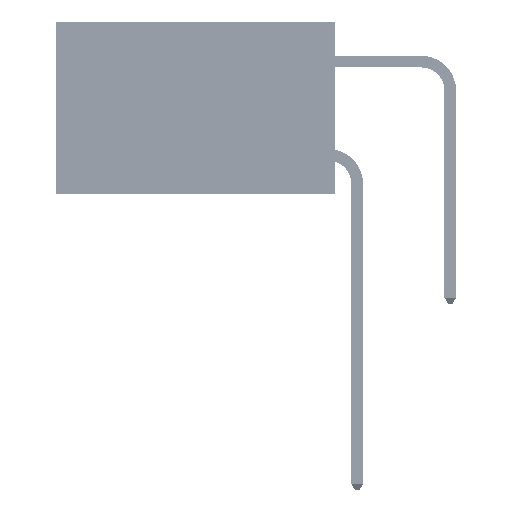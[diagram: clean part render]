
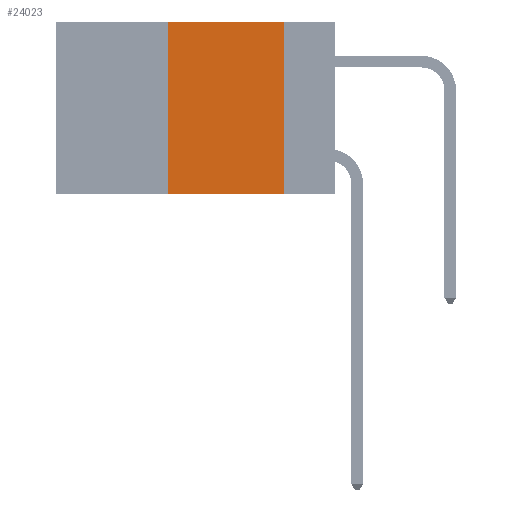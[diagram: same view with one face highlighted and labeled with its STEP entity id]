
A CAD part, left-side view. The second image highlights one B-rep face of the part: STEP entity #24023.
In plain terms, the highlighted planar face has unit normal (-1, 0, 0).
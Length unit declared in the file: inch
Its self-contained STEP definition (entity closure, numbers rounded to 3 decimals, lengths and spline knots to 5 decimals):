
#406 = CARTESIAN_POINT ( 'NONE',  ( 0., 0.11, -0.37 ) ) ;
#1248 = LINE ( 'NONE', #21266, #43485 ) ;
#2082 = EDGE_CURVE ( 'NONE', #16525, #44125, #23663, .T. ) ;
#4859 = VERTEX_POINT ( 'NONE', #8929 ) ;
#5444 = CARTESIAN_POINT ( 'NONE',  ( 0., 0.6, -0.37 ) ) ;
#6294 = VECTOR ( 'NONE', #39252, 39.37008 ) ;
#7403 = VECTOR ( 'NONE', #13469, 39.37008 ) ;
#8119 = ORIENTED_EDGE ( 'NONE', *, *, #2082, .F. ) ;
#8929 = CARTESIAN_POINT ( 'NONE',  ( 0., 0.36, -0.37 ) ) ;
#13469 = DIRECTION ( 'NONE',  ( 0., -1., 0. ) ) ;
#15830 = EDGE_CURVE ( 'NONE', #4859, #45091, #19500, .T. ) ;
#16202 = ORIENTED_EDGE ( 'NONE', *, *, #34832, .T. ) ;
#16525 = VERTEX_POINT ( 'NONE', #41664 ) ;
#17054 = CARTESIAN_POINT ( 'NONE',  ( 0., 0.36, 0. ) ) ;
#19500 = LINE ( 'NONE', #20478, #6294 ) ;
#20478 = CARTESIAN_POINT ( 'NONE',  ( 0., 0.36, 0. ) ) ;
#21266 = CARTESIAN_POINT ( 'NONE',  ( 0., 0.6, 0. ) ) ;
#21524 = FACE_OUTER_BOUND ( 'NONE', #23746, .T. ) ;
#23663 = LINE ( 'NONE', #42945, #49479 ) ;
#23746 = EDGE_LOOP ( 'NONE', ( #8119, #33545, #30212, #16202 ) ) ;
#23912 = DIRECTION ( 'NONE',  ( 0., 0., -1. ) ) ;
#24023 = ADVANCED_FACE ( 'NONE', ( #21524 ), #29278, .F. ) ;
#24230 = LINE ( 'NONE', #5444, #7403 ) ;
#25772 = CARTESIAN_POINT ( 'NONE',  ( 0., 0.6, 0. ) ) ;
#29011 = DIRECTION ( 'NONE',  ( 0., -1., 0. ) ) ;
#29027 = DIRECTION ( 'NONE',  ( 1., 0., 0. ) ) ;
#29278 = PLANE ( 'NONE',  #29699 ) ;
#29699 = AXIS2_PLACEMENT_3D ( 'NONE', #25772, #29027, #33020 ) ;
#30212 = ORIENTED_EDGE ( 'NONE', *, *, #15830, .F. ) ;
#33020 = DIRECTION ( 'NONE',  ( 0., 0., -1. ) ) ;
#33545 = ORIENTED_EDGE ( 'NONE', *, *, #37646, .F. ) ;
#34832 = EDGE_CURVE ( 'NONE', #4859, #44125, #24230, .T. ) ;
#37646 = EDGE_CURVE ( 'NONE', #45091, #16525, #1248, .T. ) ;
#39252 = DIRECTION ( 'NONE',  ( 0., 0., 1. ) ) ;
#41664 = CARTESIAN_POINT ( 'NONE',  ( 0., 0.11, 0. ) ) ;
#42945 = CARTESIAN_POINT ( 'NONE',  ( 0., 0.11, 0. ) ) ;
#43485 = VECTOR ( 'NONE', #29011, 39.37008 ) ;
#44125 = VERTEX_POINT ( 'NONE', #406 ) ;
#45091 = VERTEX_POINT ( 'NONE', #17054 ) ;
#49479 = VECTOR ( 'NONE', #23912, 39.37008 ) ;
